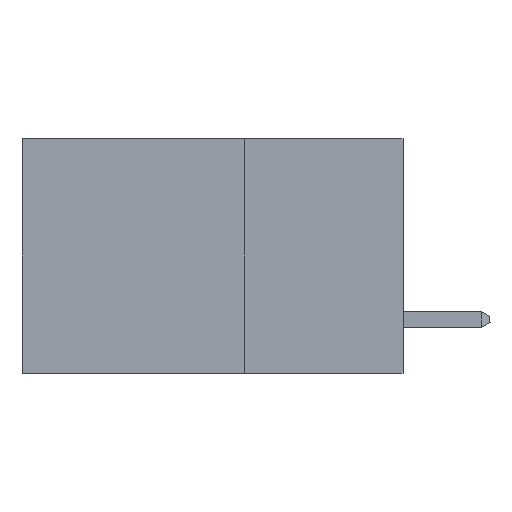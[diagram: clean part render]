
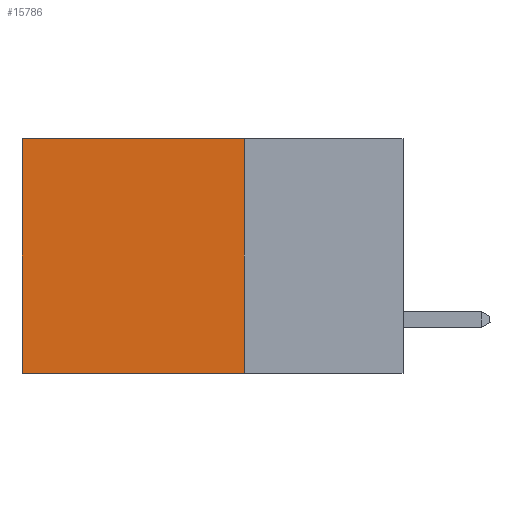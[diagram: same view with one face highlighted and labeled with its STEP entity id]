
A CAD part, left-side view. The second image highlights one B-rep face of the part: STEP entity #15786.
In plain terms, the highlighted planar face has unit normal (-1, 0, 0).
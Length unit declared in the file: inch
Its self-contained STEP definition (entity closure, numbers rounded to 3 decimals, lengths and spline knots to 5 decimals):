
#884 = CARTESIAN_POINT ( 'NONE',  ( 0.2875, 0.25, 0. ) ) ;
#1352 = EDGE_CURVE ( 'NONE', #33741, #17977, #34369, .T. ) ;
#2584 = VECTOR ( 'NONE', #41512, 39.37008 ) ;
#2803 = ORIENTED_EDGE ( 'NONE', *, *, #1352, .F. ) ;
#7520 = CARTESIAN_POINT ( 'NONE',  ( 0.2875, 0.25, 0. ) ) ;
#7811 = DIRECTION ( 'NONE',  ( 0., 1., 0. ) ) ;
#8212 = CARTESIAN_POINT ( 'NONE',  ( 0.2875, 0.25, 0. ) ) ;
#8852 = DIRECTION ( 'NONE',  ( 1., 0., 0. ) ) ;
#9006 = DIRECTION ( 'NONE',  ( 0., 0., -1. ) ) ;
#9537 = AXIS2_PLACEMENT_3D ( 'NONE', #23024, #8852, #9006 ) ;
#11479 = CARTESIAN_POINT ( 'NONE',  ( 0.2875, 0.6, 0. ) ) ;
#11711 = VERTEX_POINT ( 'NONE', #35066 ) ;
#13218 = ORIENTED_EDGE ( 'NONE', *, *, #42748, .F. ) ;
#13585 = VECTOR ( 'NONE', #7811, 39.37008 ) ;
#15786 = ADVANCED_FACE ( 'NONE', ( #18467 ), #19533, .F. ) ;
#17977 = VERTEX_POINT ( 'NONE', #21835 ) ;
#18467 = FACE_OUTER_BOUND ( 'NONE', #41426, .T. ) ;
#19533 = PLANE ( 'NONE',  #9537 ) ;
#20025 = ORIENTED_EDGE ( 'NONE', *, *, #21282, .T. ) ;
#21282 = EDGE_CURVE ( 'NONE', #33741, #41093, #24856, .T. ) ;
#21294 = LINE ( 'NONE', #11479, #29392 ) ;
#21835 = CARTESIAN_POINT ( 'NONE',  ( 0.2875, 0.25, -0.37 ) ) ;
#23024 = CARTESIAN_POINT ( 'NONE',  ( 0.2875, 0.25, 0. ) ) ;
#24856 = LINE ( 'NONE', #884, #13585 ) ;
#28890 = DIRECTION ( 'NONE',  ( 0., 1., 0. ) ) ;
#29050 = EDGE_CURVE ( 'NONE', #41093, #11711, #21294, .T. ) ;
#29392 = VECTOR ( 'NONE', #32509, 39.37008 ) ;
#32509 = DIRECTION ( 'NONE',  ( 0., 0., -1. ) ) ;
#33091 = CARTESIAN_POINT ( 'NONE',  ( 0.2875, 0.6, 0. ) ) ;
#33741 = VERTEX_POINT ( 'NONE', #8212 ) ;
#34369 = LINE ( 'NONE', #7520, #2584 ) ;
#35066 = CARTESIAN_POINT ( 'NONE',  ( 0.2875, 0.6, -0.37 ) ) ;
#35965 = CARTESIAN_POINT ( 'NONE',  ( 0.2875, 0.25, -0.37 ) ) ;
#37571 = LINE ( 'NONE', #35965, #44019 ) ;
#41093 = VERTEX_POINT ( 'NONE', #33091 ) ;
#41426 = EDGE_LOOP ( 'NONE', ( #43947, #13218, #2803, #20025 ) ) ;
#41512 = DIRECTION ( 'NONE',  ( 0., 0., -1. ) ) ;
#42748 = EDGE_CURVE ( 'NONE', #17977, #11711, #37571, .T. ) ;
#43947 = ORIENTED_EDGE ( 'NONE', *, *, #29050, .T. ) ;
#44019 = VECTOR ( 'NONE', #28890, 39.37008 ) ;
